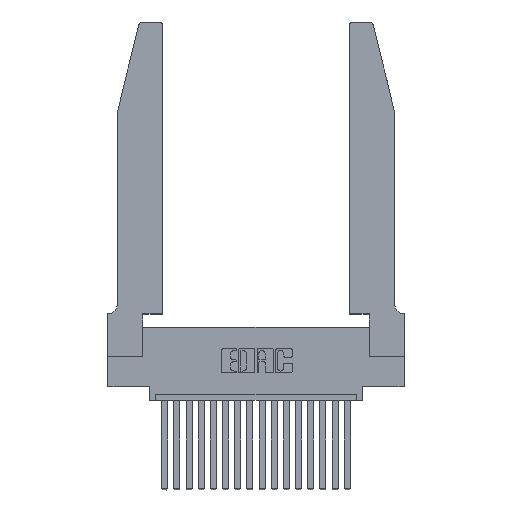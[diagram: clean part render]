
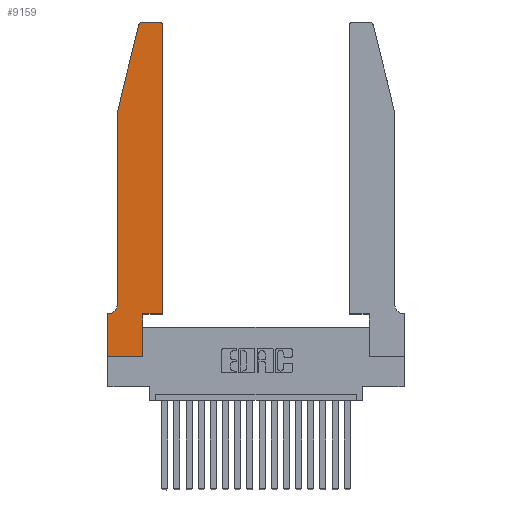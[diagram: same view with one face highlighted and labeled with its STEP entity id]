
A CAD part, top view. The second image highlights one B-rep face of the part: STEP entity #9159.
In plain terms, the highlighted planar face has unit normal (0, 0, 1).
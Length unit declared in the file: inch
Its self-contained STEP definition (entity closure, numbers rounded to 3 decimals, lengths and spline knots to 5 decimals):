
#239 = AXIS2_PLACEMENT_3D ( 'NONE', #17993, #916, #4222 ) ;
#619 = VECTOR ( 'NONE', #9908, 39.37008 ) ;
#916 = DIRECTION ( 'NONE',  ( 0., 0., 1. ) ) ;
#1001 = VERTEX_POINT ( 'NONE', #18656 ) ;
#1207 = DIRECTION ( 'NONE',  ( 0., 0., 1. ) ) ;
#1327 = CARTESIAN_POINT ( 'NONE',  ( 0.2865, 0.35, 0.37 ) ) ;
#1356 = LINE ( 'NONE', #7084, #15313 ) ;
#1578 = VERTEX_POINT ( 'NONE', #5003 ) ;
#1586 = CARTESIAN_POINT ( 'NONE',  ( 0., 0.35, 0.37 ) ) ;
#1812 = VERTEX_POINT ( 'NONE', #18077 ) ;
#2144 = AXIS2_PLACEMENT_3D ( 'NONE', #1586, #9280, #20176 ) ;
#2440 = DIRECTION ( 'NONE',  ( -0.239, -0.971, 0. ) ) ;
#2518 = EDGE_CURVE ( 'NONE', #1001, #15487, #11463, .T. ) ;
#2773 = EDGE_CURVE ( 'NONE', #15487, #7928, #3899, .T. ) ;
#2836 = DIRECTION ( 'NONE',  ( 0., -1., 0. ) ) ;
#2894 = VERTEX_POINT ( 'NONE', #8465 ) ;
#2947 = VECTOR ( 'NONE', #2836, 39.37008 ) ;
#3397 = CIRCLE ( 'NONE', #239, 0.03 ) ;
#3832 = CARTESIAN_POINT ( 'NONE',  ( 0.2605, 2.75, 0.37 ) ) ;
#3885 = VECTOR ( 'NONE', #16948, 39.37008 ) ;
#3899 = CIRCLE ( 'NONE', #16854, 0.07 ) ;
#4222 = DIRECTION ( 'NONE',  ( 1., 0., 0. ) ) ;
#4495 = VERTEX_POINT ( 'NONE', #20096 ) ;
#4584 = CARTESIAN_POINT ( 'NONE',  ( 0.0055, 0.42, 0.37 ) ) ;
#4671 = ORIENTED_EDGE ( 'NONE', *, *, #11125, .T. ) ;
#5003 = CARTESIAN_POINT ( 'NONE',  ( 0.4205, 2.75, 0.37 ) ) ;
#5566 = CARTESIAN_POINT ( 'NONE',  ( 0.0755, 0.35, 0.37 ) ) ;
#5588 = VECTOR ( 'NONE', #17040, 39.37008 ) ;
#5702 = EDGE_CURVE ( 'NONE', #14386, #4495, #7964, .T. ) ;
#5774 = EDGE_CURVE ( 'NONE', #1812, #1001, #1356, .T. ) ;
#6301 = CARTESIAN_POINT ( 'NONE',  ( 0., 0.35, 0.37 ) ) ;
#6695 = CARTESIAN_POINT ( 'NONE',  ( 0.4505, 0.35, 0.37 ) ) ;
#7045 = CARTESIAN_POINT ( 'NONE',  ( 0.0755, 2., 0.37 ) ) ;
#7084 = CARTESIAN_POINT ( 'NONE',  ( 0.0755, 2., 0.37 ) ) ;
#7248 = CARTESIAN_POINT ( 'NONE',  ( 0.4505, 0.35, 0.37 ) ) ;
#7307 = DIRECTION ( 'NONE',  ( 0., -1., 0. ) ) ;
#7700 = LINE ( 'NONE', #5566, #10873 ) ;
#7928 = VERTEX_POINT ( 'NONE', #15729 ) ;
#7964 = LINE ( 'NONE', #6695, #619 ) ;
#8465 = CARTESIAN_POINT ( 'NONE',  ( 0.2865, 0.35, 0.37 ) ) ;
#8718 = CARTESIAN_POINT ( 'NONE',  ( 0.4505, 0.35, 0.37 ) ) ;
#8901 = ORIENTED_EDGE ( 'NONE', *, *, #13576, .T. ) ;
#8968 = CARTESIAN_POINT ( 'NONE',  ( 0.2865, 0., 0.37 ) ) ;
#9159 = ADVANCED_FACE ( 'NONE', ( #18807 ), #10974, .T. ) ;
#9280 = DIRECTION ( 'NONE',  ( 0., 0., 1. ) ) ;
#9315 = ORIENTED_EDGE ( 'NONE', *, *, #5702, .T. ) ;
#9455 = LINE ( 'NONE', #3832, #12868 ) ;
#9870 = ORIENTED_EDGE ( 'NONE', *, *, #5774, .T. ) ;
#9908 = DIRECTION ( 'NONE',  ( 0., 1., 0. ) ) ;
#9919 = ORIENTED_EDGE ( 'NONE', *, *, #2518, .T. ) ;
#9992 = VECTOR ( 'NONE', #13437, 39.37008 ) ;
#10241 = LINE ( 'NONE', #12500, #5588 ) ;
#10390 = ORIENTED_EDGE ( 'NONE', *, *, #10427, .T. ) ;
#10427 = EDGE_CURVE ( 'NONE', #17246, #18639, #17573, .T. ) ;
#10565 = CARTESIAN_POINT ( 'NONE',  ( 0.284, 2.72, 0.37 ) ) ;
#10873 = VECTOR ( 'NONE', #19730, 39.37008 ) ;
#10974 = PLANE ( 'NONE',  #2144 ) ;
#11080 = EDGE_CURVE ( 'NONE', #4495, #1578, #3397, .T. ) ;
#11125 = EDGE_CURVE ( 'NONE', #2894, #14386, #12190, .T. ) ;
#11261 = EDGE_CURVE ( 'NONE', #14467, #2894, #14638, .T. ) ;
#11463 = LINE ( 'NONE', #7045, #14910 ) ;
#11593 = CARTESIAN_POINT ( 'NONE',  ( 0.0755, 0.42, 0.37 ) ) ;
#11662 = DIRECTION ( 'NONE',  ( -1., 0., 0. ) ) ;
#12048 = ORIENTED_EDGE ( 'NONE', *, *, #17929, .T. ) ;
#12156 = DIRECTION ( 'NONE',  ( 1., 0., 0. ) ) ;
#12190 = LINE ( 'NONE', #8718, #9992 ) ;
#12272 = CIRCLE ( 'NONE', #14984, 0.03 ) ;
#12438 = VERTEX_POINT ( 'NONE', #13579 ) ;
#12439 = DIRECTION ( 'NONE',  ( -1., 0., 0. ) ) ;
#12500 = CARTESIAN_POINT ( 'NONE',  ( 0., 0., 0.37 ) ) ;
#12672 = CARTESIAN_POINT ( 'NONE',  ( 0., 0., 0.37 ) ) ;
#12868 = VECTOR ( 'NONE', #11662, 39.37008 ) ;
#13437 = DIRECTION ( 'NONE',  ( 1., 0., 0. ) ) ;
#13576 = EDGE_CURVE ( 'NONE', #1578, #12438, #9455, .T. ) ;
#13579 = CARTESIAN_POINT ( 'NONE',  ( 0.284, 2.75, 0.37 ) ) ;
#14386 = VERTEX_POINT ( 'NONE', #7248 ) ;
#14467 = VERTEX_POINT ( 'NONE', #8968 ) ;
#14638 = LINE ( 'NONE', #1327, #3885 ) ;
#14660 = ORIENTED_EDGE ( 'NONE', *, *, #11261, .T. ) ;
#14666 = ORIENTED_EDGE ( 'NONE', *, *, #2773, .T. ) ;
#14910 = VECTOR ( 'NONE', #7307, 39.37008 ) ;
#14984 = AXIS2_PLACEMENT_3D ( 'NONE', #10565, #1207, #12156 ) ;
#15018 = ORIENTED_EDGE ( 'NONE', *, *, #16524, .T. ) ;
#15028 = EDGE_LOOP ( 'NONE', ( #8901, #15018, #9870, #9919, #14666, #16688, #10390, #12048, #14660, #4671, #9315, #15822 ) ) ;
#15313 = VECTOR ( 'NONE', #2440, 39.37008 ) ;
#15487 = VERTEX_POINT ( 'NONE', #11593 ) ;
#15546 = CARTESIAN_POINT ( 'NONE',  ( 0., 0., 0.37 ) ) ;
#15702 = DIRECTION ( 'NONE',  ( 0., 0., -1. ) ) ;
#15729 = CARTESIAN_POINT ( 'NONE',  ( 0.0055, 0.35, 0.37 ) ) ;
#15822 = ORIENTED_EDGE ( 'NONE', *, *, #11080, .T. ) ;
#16524 = EDGE_CURVE ( 'NONE', #12438, #1812, #12272, .T. ) ;
#16688 = ORIENTED_EDGE ( 'NONE', *, *, #20235, .T. ) ;
#16854 = AXIS2_PLACEMENT_3D ( 'NONE', #4584, #15702, #12439 ) ;
#16948 = DIRECTION ( 'NONE',  ( 0., 1., 0. ) ) ;
#17040 = DIRECTION ( 'NONE',  ( 1., 0., 0. ) ) ;
#17246 = VERTEX_POINT ( 'NONE', #6301 ) ;
#17573 = LINE ( 'NONE', #15546, #2947 ) ;
#17929 = EDGE_CURVE ( 'NONE', #18639, #14467, #10241, .T. ) ;
#17993 = CARTESIAN_POINT ( 'NONE',  ( 0.4205, 2.72, 0.37 ) ) ;
#18077 = CARTESIAN_POINT ( 'NONE',  ( 0.25487, 2.72718, 0.37 ) ) ;
#18639 = VERTEX_POINT ( 'NONE', #12672 ) ;
#18656 = CARTESIAN_POINT ( 'NONE',  ( 0.0755, 2., 0.37 ) ) ;
#18807 = FACE_OUTER_BOUND ( 'NONE', #15028, .T. ) ;
#19730 = DIRECTION ( 'NONE',  ( -1., 0., 0. ) ) ;
#20096 = CARTESIAN_POINT ( 'NONE',  ( 0.4505, 2.72, 0.37 ) ) ;
#20176 = DIRECTION ( 'NONE',  ( 1., 0., 0. ) ) ;
#20235 = EDGE_CURVE ( 'NONE', #7928, #17246, #7700, .T. ) ;
